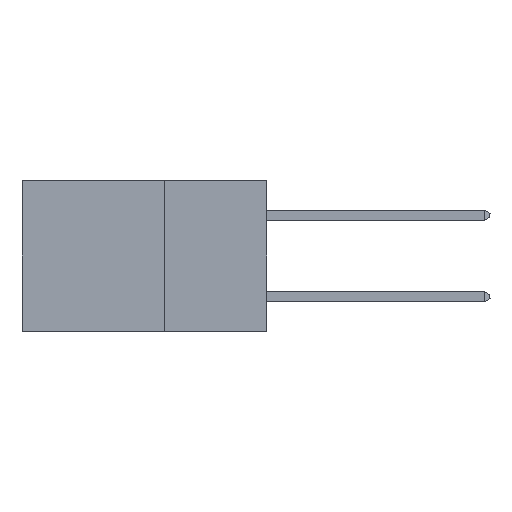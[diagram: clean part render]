
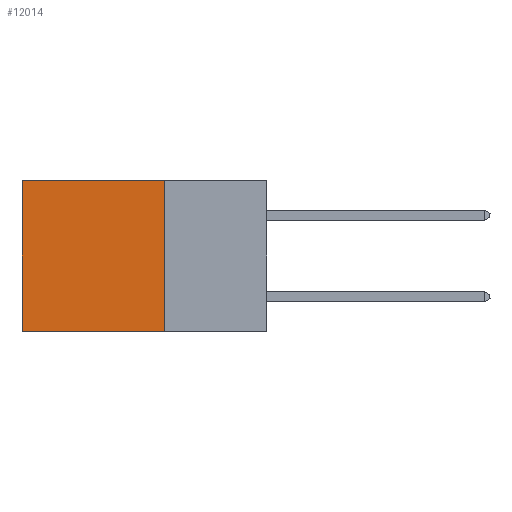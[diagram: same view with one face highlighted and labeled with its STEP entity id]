
A CAD part, left-side view. The second image highlights one B-rep face of the part: STEP entity #12014.
In plain terms, the highlighted planar face has unit normal (-1, 0, 0).
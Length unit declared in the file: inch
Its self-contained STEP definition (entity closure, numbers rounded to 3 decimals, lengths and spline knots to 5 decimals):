
#135 = VECTOR ( 'NONE', #15042, 39.37008 ) ;
#1326 = CARTESIAN_POINT ( 'NONE',  ( 0.2875, 0.25, -0.37 ) ) ;
#1891 = PLANE ( 'NONE',  #20499 ) ;
#2058 = LINE ( 'NONE', #7444, #16046 ) ;
#3181 = VERTEX_POINT ( 'NONE', #17283 ) ;
#3612 = EDGE_CURVE ( 'NONE', #6279, #16799, #2058, .T. ) ;
#3743 = EDGE_LOOP ( 'NONE', ( #16774, #11288, #15828, #9284 ) ) ;
#5286 = EDGE_CURVE ( 'NONE', #15762, #3181, #21256, .T. ) ;
#5354 = DIRECTION ( 'NONE',  ( 0., 0., -1. ) ) ;
#6279 = VERTEX_POINT ( 'NONE', #6942 ) ;
#6942 = CARTESIAN_POINT ( 'NONE',  ( 0.2875, 0.25, 0. ) ) ;
#7029 = CARTESIAN_POINT ( 'NONE',  ( 0.2875, 0.25, 0. ) ) ;
#7359 = EDGE_CURVE ( 'NONE', #16799, #3181, #14956, .T. ) ;
#7444 = CARTESIAN_POINT ( 'NONE',  ( 0.2875, 0.25, 0. ) ) ;
#8402 = DIRECTION ( 'NONE',  ( 1., 0., 0. ) ) ;
#8691 = FACE_OUTER_BOUND ( 'NONE', #3743, .T. ) ;
#9284 = ORIENTED_EDGE ( 'NONE', *, *, #12490, .T. ) ;
#10629 = DIRECTION ( 'NONE',  ( 0., 1., 0. ) ) ;
#11288 = ORIENTED_EDGE ( 'NONE', *, *, #7359, .F. ) ;
#12014 = ADVANCED_FACE ( 'NONE', ( #8691 ), #1891, .F. ) ;
#12490 = EDGE_CURVE ( 'NONE', #6279, #15762, #17924, .T. ) ;
#13351 = VECTOR ( 'NONE', #10629, 39.37008 ) ;
#14956 = LINE ( 'NONE', #15301, #13351 ) ;
#14962 = CARTESIAN_POINT ( 'NONE',  ( 0.2875, 0.6, 0. ) ) ;
#15041 = CARTESIAN_POINT ( 'NONE',  ( 0.2875, 0.25, 0. ) ) ;
#15042 = DIRECTION ( 'NONE',  ( 0., 0., -1. ) ) ;
#15301 = CARTESIAN_POINT ( 'NONE',  ( 0.2875, 0.25, -0.37 ) ) ;
#15762 = VERTEX_POINT ( 'NONE', #14962 ) ;
#15828 = ORIENTED_EDGE ( 'NONE', *, *, #3612, .F. ) ;
#16046 = VECTOR ( 'NONE', #19447, 39.37008 ) ;
#16774 = ORIENTED_EDGE ( 'NONE', *, *, #5286, .T. ) ;
#16799 = VERTEX_POINT ( 'NONE', #1326 ) ;
#17283 = CARTESIAN_POINT ( 'NONE',  ( 0.2875, 0.6, -0.37 ) ) ;
#17924 = LINE ( 'NONE', #15041, #20554 ) ;
#19447 = DIRECTION ( 'NONE',  ( 0., 0., -1. ) ) ;
#19939 = DIRECTION ( 'NONE',  ( 0., 1., 0. ) ) ;
#20073 = CARTESIAN_POINT ( 'NONE',  ( 0.2875, 0.6, 0. ) ) ;
#20499 = AXIS2_PLACEMENT_3D ( 'NONE', #7029, #8402, #5354 ) ;
#20554 = VECTOR ( 'NONE', #19939, 39.37008 ) ;
#21256 = LINE ( 'NONE', #20073, #135 ) ;
